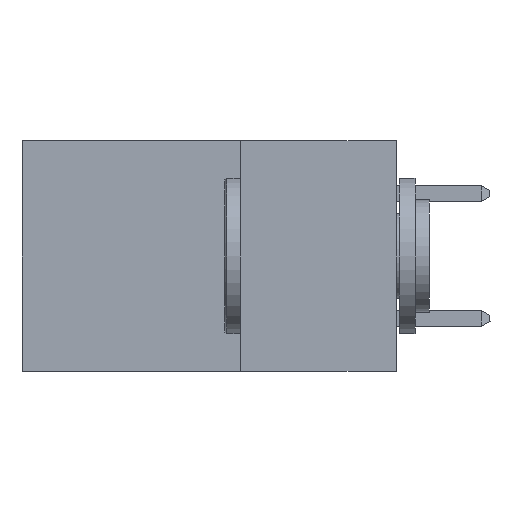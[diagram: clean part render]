
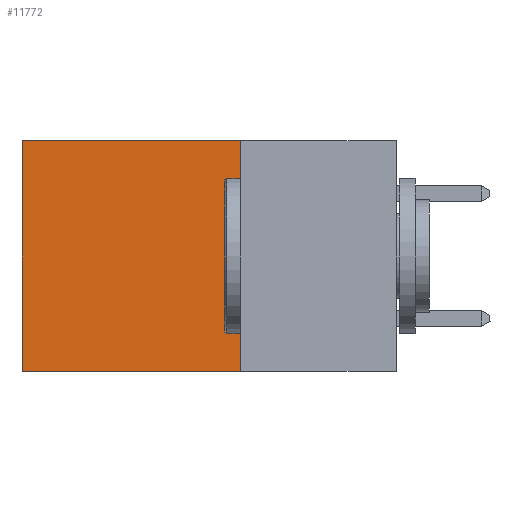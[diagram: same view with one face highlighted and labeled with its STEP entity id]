
A CAD part, left-side view. The second image highlights one B-rep face of the part: STEP entity #11772.
In plain terms, the highlighted planar face has unit normal (-1, 0, 0).
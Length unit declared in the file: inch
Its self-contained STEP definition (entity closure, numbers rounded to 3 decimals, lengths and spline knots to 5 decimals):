
#176 = ORIENTED_EDGE ( 'NONE', *, *, #2337, .T. ) ;
#1203 = AXIS2_PLACEMENT_3D ( 'NONE', #1376, #10284, #25519 ) ;
#1376 = CARTESIAN_POINT ( 'NONE',  ( 0.2615, 0.25, -0.37 ) ) ;
#2337 = EDGE_CURVE ( 'NONE', #10977, #5835, #23428, .T. ) ;
#2762 = ORIENTED_EDGE ( 'NONE', *, *, #19771, .F. ) ;
#2821 = VECTOR ( 'NONE', #27578, 39.37008 ) ;
#2916 = CARTESIAN_POINT ( 'NONE',  ( 0.2615, 0.6, 0. ) ) ;
#3851 = CARTESIAN_POINT ( 'NONE',  ( 0.2615, 0.6, -0.37 ) ) ;
#5634 = ORIENTED_EDGE ( 'NONE', *, *, #8982, .F. ) ;
#5835 = VERTEX_POINT ( 'NONE', #15879 ) ;
#5920 = VECTOR ( 'NONE', #19307, 39.37008 ) ;
#6485 = VECTOR ( 'NONE', #27113, 39.37008 ) ;
#7593 = CARTESIAN_POINT ( 'NONE',  ( 0.2615, 0.25, 0. ) ) ;
#7971 = VERTEX_POINT ( 'NONE', #18742 ) ;
#8051 = LINE ( 'NONE', #25456, #2821 ) ;
#8982 = EDGE_CURVE ( 'NONE', #14767, #5835, #8051, .T. ) ;
#10284 = DIRECTION ( 'NONE',  ( 1., 0., 0. ) ) ;
#10977 = VERTEX_POINT ( 'NONE', #2916 ) ;
#11772 = ADVANCED_FACE ( 'NONE', ( #12428 ), #16872, .F. ) ;
#12425 = LINE ( 'NONE', #7593, #6485 ) ;
#12428 = FACE_OUTER_BOUND ( 'NONE', #27484, .T. ) ;
#13605 = VECTOR ( 'NONE', #19862, 39.37008 ) ;
#14299 = LINE ( 'NONE', #17702, #13605 ) ;
#14767 = VERTEX_POINT ( 'NONE', #26368 ) ;
#15879 = CARTESIAN_POINT ( 'NONE',  ( 0.2615, 0.6, -0.37 ) ) ;
#16872 = PLANE ( 'NONE',  #1203 ) ;
#17702 = CARTESIAN_POINT ( 'NONE',  ( 0.2615, 0.25, -0.37 ) ) ;
#18742 = CARTESIAN_POINT ( 'NONE',  ( 0.2615, 0.25, 0. ) ) ;
#19307 = DIRECTION ( 'NONE',  ( 0., 0., -1. ) ) ;
#19771 = EDGE_CURVE ( 'NONE', #7971, #14767, #14299, .T. ) ;
#19862 = DIRECTION ( 'NONE',  ( 0., 0., -1. ) ) ;
#23428 = LINE ( 'NONE', #3851, #5920 ) ;
#25456 = CARTESIAN_POINT ( 'NONE',  ( 0.2615, 0.25, -0.37 ) ) ;
#25519 = DIRECTION ( 'NONE',  ( 0., 0., -1. ) ) ;
#26326 = EDGE_CURVE ( 'NONE', #7971, #10977, #12425, .T. ) ;
#26368 = CARTESIAN_POINT ( 'NONE',  ( 0.2615, 0.25, -0.37 ) ) ;
#27113 = DIRECTION ( 'NONE',  ( 0., 1., 0. ) ) ;
#27306 = ORIENTED_EDGE ( 'NONE', *, *, #26326, .T. ) ;
#27484 = EDGE_LOOP ( 'NONE', ( #176, #5634, #2762, #27306 ) ) ;
#27578 = DIRECTION ( 'NONE',  ( 0., 1., 0. ) ) ;
